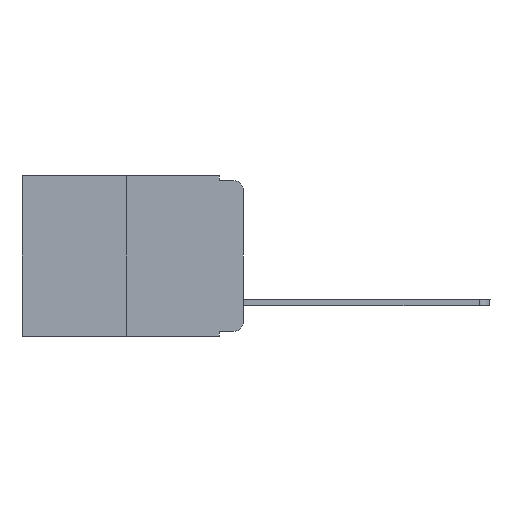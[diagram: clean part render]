
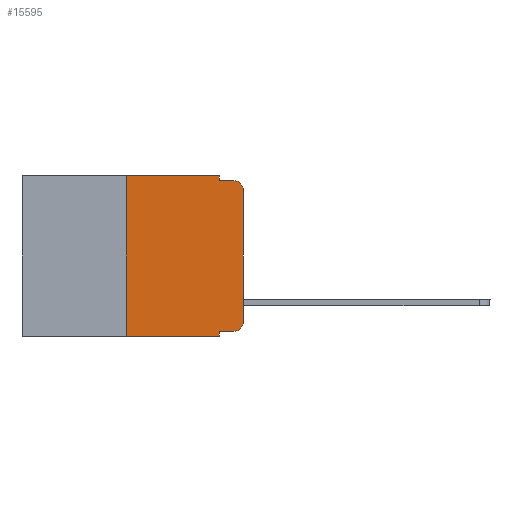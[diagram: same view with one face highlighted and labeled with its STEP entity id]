
A CAD part, left-side view. The second image highlights one B-rep face of the part: STEP entity #15595.
In plain terms, the highlighted planar face has unit normal (-1, 0, 0).
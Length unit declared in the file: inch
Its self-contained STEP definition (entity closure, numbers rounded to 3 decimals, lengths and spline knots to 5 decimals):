
#90 = EDGE_CURVE ( 'NONE', #12661, #12442, #14681, .T. ) ;
#588 = ORIENTED_EDGE ( 'NONE', *, *, #90, .F. ) ;
#1033 = CARTESIAN_POINT ( 'NONE',  ( 0., 0.25, 0. ) ) ;
#1179 = CARTESIAN_POINT ( 'NONE',  ( 0., 0., -0.03 ) ) ;
#1947 = ORIENTED_EDGE ( 'NONE', *, *, #6614, .T. ) ;
#2028 = DIRECTION ( 'NONE',  ( 0., 0., 1. ) ) ;
#2031 = VERTEX_POINT ( 'NONE', #21056 ) ;
#2058 = VECTOR ( 'NONE', #13864, 39.37008 ) ;
#2061 = DIRECTION ( 'NONE',  ( -1., 0., 0. ) ) ;
#2131 = FACE_OUTER_BOUND ( 'NONE', #10496, .T. ) ;
#2455 = CARTESIAN_POINT ( 'NONE',  ( 0., 0.051, -0.333 ) ) ;
#2542 = EDGE_CURVE ( 'NONE', #7777, #11252, #22311, .T. ) ;
#3223 = EDGE_CURVE ( 'NONE', #20372, #12442, #17198, .T. ) ;
#3637 = LINE ( 'NONE', #17340, #16685 ) ;
#3648 = LINE ( 'NONE', #5158, #12382 ) ;
#3728 = CARTESIAN_POINT ( 'NONE',  ( 0., 0.473, 0. ) ) ;
#3776 = CARTESIAN_POINT ( 'NONE',  ( 0., 0.02, -0.313 ) ) ;
#3865 = ORIENTED_EDGE ( 'NONE', *, *, #2542, .T. ) ;
#3997 = CARTESIAN_POINT ( 'NONE',  ( 0., 0.25, 0. ) ) ;
#4174 = DIRECTION ( 'NONE',  ( 0., 0., -1. ) ) ;
#4243 = CARTESIAN_POINT ( 'NONE',  ( 0., 0.051, -0.01 ) ) ;
#4352 = EDGE_CURVE ( 'NONE', #20372, #20163, #5729, .T. ) ;
#4603 = ORIENTED_EDGE ( 'NONE', *, *, #14955, .F. ) ;
#4868 = CARTESIAN_POINT ( 'NONE',  ( 0., 0.051, -0.343 ) ) ;
#5158 = CARTESIAN_POINT ( 'NONE',  ( 0., 0., 0. ) ) ;
#5357 = DIRECTION ( 'NONE',  ( 0., 0., -1. ) ) ;
#5729 = LINE ( 'NONE', #3997, #20483 ) ;
#6614 = EDGE_CURVE ( 'NONE', #12661, #7777, #15357, .T. ) ;
#6706 = ORIENTED_EDGE ( 'NONE', *, *, #17276, .F. ) ;
#6971 = DIRECTION ( 'NONE',  ( 1., 0., 0. ) ) ;
#7292 = LINE ( 'NONE', #9139, #16702 ) ;
#7767 = ORIENTED_EDGE ( 'NONE', *, *, #8719, .T. ) ;
#7777 = VERTEX_POINT ( 'NONE', #21946 ) ;
#8269 = CIRCLE ( 'NONE', #14167, 0.02 ) ;
#8719 = EDGE_CURVE ( 'NONE', #11252, #21087, #3648, .T. ) ;
#8800 = CARTESIAN_POINT ( 'NONE',  ( 0., 0.473, 0. ) ) ;
#9139 = CARTESIAN_POINT ( 'NONE',  ( 0., 0.051, 0. ) ) ;
#9446 = VERTEX_POINT ( 'NONE', #9862 ) ;
#9840 = EDGE_CURVE ( 'NONE', #21087, #9446, #8269, .T. ) ;
#9862 = CARTESIAN_POINT ( 'NONE',  ( 0., 0.02, -0.01 ) ) ;
#10178 = VECTOR ( 'NONE', #13736, 39.37008 ) ;
#10496 = EDGE_LOOP ( 'NONE', ( #7767, #22107, #15884, #4603, #6706, #13642, #22216, #588, #1947, #3865 ) ) ;
#11046 = VECTOR ( 'NONE', #4174, 39.37008 ) ;
#11252 = VERTEX_POINT ( 'NONE', #19671 ) ;
#12256 = CARTESIAN_POINT ( 'NONE',  ( 0., 0.473, -0.343 ) ) ;
#12382 = VECTOR ( 'NONE', #2028, 39.37008 ) ;
#12389 = LINE ( 'NONE', #8800, #13496 ) ;
#12442 = VERTEX_POINT ( 'NONE', #4868 ) ;
#12545 = DIRECTION ( 'NONE',  ( 0., -1., 0. ) ) ;
#12661 = VERTEX_POINT ( 'NONE', #2455 ) ;
#13175 = AXIS2_PLACEMENT_3D ( 'NONE', #3776, #2061, #16127 ) ;
#13230 = EDGE_CURVE ( 'NONE', #21883, #9446, #3637, .T. ) ;
#13496 = VECTOR ( 'NONE', #17880, 39.37008 ) ;
#13642 = ORIENTED_EDGE ( 'NONE', *, *, #4352, .F. ) ;
#13736 = DIRECTION ( 'NONE',  ( 0., -1., 0. ) ) ;
#13864 = DIRECTION ( 'NONE',  ( 0., -1., 0. ) ) ;
#14167 = AXIS2_PLACEMENT_3D ( 'NONE', #19625, #15665, #17270 ) ;
#14681 = LINE ( 'NONE', #18223, #11046 ) ;
#14955 = EDGE_CURVE ( 'NONE', #2031, #21883, #7292, .T. ) ;
#15357 = LINE ( 'NONE', #22573, #2058 ) ;
#15595 = ADVANCED_FACE ( 'NONE', ( #2131 ), #21097, .F. ) ;
#15665 = DIRECTION ( 'NONE',  ( -1., 0., 0. ) ) ;
#15884 = ORIENTED_EDGE ( 'NONE', *, *, #13230, .F. ) ;
#16127 = DIRECTION ( 'NONE',  ( 0., 0., -1. ) ) ;
#16685 = VECTOR ( 'NONE', #12545, 39.37008 ) ;
#16702 = VECTOR ( 'NONE', #18332, 39.37008 ) ;
#17198 = LINE ( 'NONE', #12256, #10178 ) ;
#17270 = DIRECTION ( 'NONE',  ( 0., 0., -1. ) ) ;
#17276 = EDGE_CURVE ( 'NONE', #20163, #2031, #12389, .T. ) ;
#17340 = CARTESIAN_POINT ( 'NONE',  ( 0., 0.051, -0.01 ) ) ;
#17880 = DIRECTION ( 'NONE',  ( 0., -1., 0. ) ) ;
#18035 = DIRECTION ( 'NONE',  ( 0., 0., 1. ) ) ;
#18223 = CARTESIAN_POINT ( 'NONE',  ( 0., 0.051, 0. ) ) ;
#18332 = DIRECTION ( 'NONE',  ( 0., 0., -1. ) ) ;
#18891 = AXIS2_PLACEMENT_3D ( 'NONE', #3728, #6971, #5357 ) ;
#19625 = CARTESIAN_POINT ( 'NONE',  ( 0., 0.02, -0.03 ) ) ;
#19671 = CARTESIAN_POINT ( 'NONE',  ( 0., 0., -0.313 ) ) ;
#20163 = VERTEX_POINT ( 'NONE', #1033 ) ;
#20372 = VERTEX_POINT ( 'NONE', #21149 ) ;
#20483 = VECTOR ( 'NONE', #18035, 39.37008 ) ;
#21056 = CARTESIAN_POINT ( 'NONE',  ( 0., 0.051, 0. ) ) ;
#21087 = VERTEX_POINT ( 'NONE', #1179 ) ;
#21097 = PLANE ( 'NONE',  #18891 ) ;
#21149 = CARTESIAN_POINT ( 'NONE',  ( 0., 0.25, -0.343 ) ) ;
#21883 = VERTEX_POINT ( 'NONE', #4243 ) ;
#21946 = CARTESIAN_POINT ( 'NONE',  ( 0., 0.02, -0.333 ) ) ;
#22107 = ORIENTED_EDGE ( 'NONE', *, *, #9840, .T. ) ;
#22216 = ORIENTED_EDGE ( 'NONE', *, *, #3223, .T. ) ;
#22311 = CIRCLE ( 'NONE', #13175, 0.02 ) ;
#22573 = CARTESIAN_POINT ( 'NONE',  ( 0., 0.051, -0.333 ) ) ;
